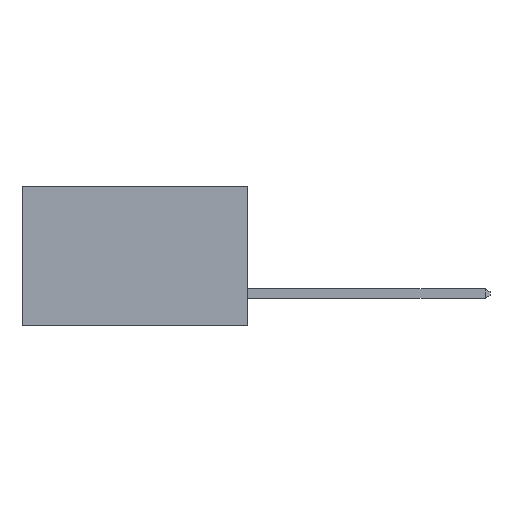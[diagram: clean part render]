
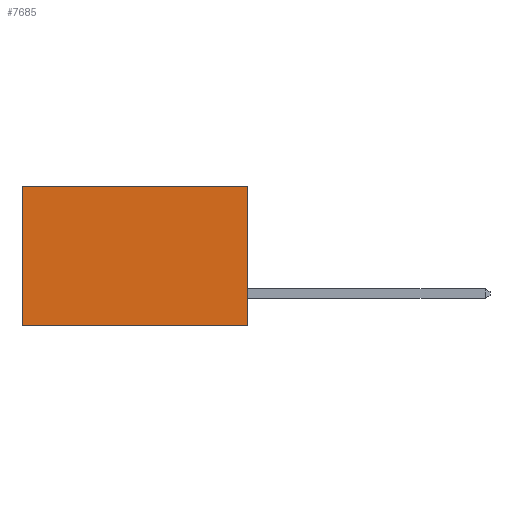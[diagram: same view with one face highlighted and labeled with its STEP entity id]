
A CAD part, left-side view. The second image highlights one B-rep face of the part: STEP entity #7685.
In plain terms, the highlighted planar face has unit normal (-1, 0, 0).
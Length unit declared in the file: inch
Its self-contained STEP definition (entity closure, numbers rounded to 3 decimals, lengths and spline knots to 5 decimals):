
#607 = VERTEX_POINT ( 'NONE', #7156 ) ;
#648 = CARTESIAN_POINT ( 'NONE',  ( 0.2615, 0., -0.37 ) ) ;
#774 = ORIENTED_EDGE ( 'NONE', *, *, #1543, .T. ) ;
#870 = VECTOR ( 'NONE', #1005, 39.37008 ) ;
#1005 = DIRECTION ( 'NONE',  ( 0., 0., -1. ) ) ;
#1362 = CARTESIAN_POINT ( 'NONE',  ( 0.2615, 0., -0.37 ) ) ;
#1461 = DIRECTION ( 'NONE',  ( 1., 0., 0. ) ) ;
#1543 = EDGE_CURVE ( 'NONE', #607, #3893, #1643, .T. ) ;
#1550 = DIRECTION ( 'NONE',  ( 0., 1., 0. ) ) ;
#1643 = LINE ( 'NONE', #3328, #7276 ) ;
#1658 = VECTOR ( 'NONE', #4089, 39.37008 ) ;
#2233 = DIRECTION ( 'NONE',  ( 0., 1., 0. ) ) ;
#2598 = ORIENTED_EDGE ( 'NONE', *, *, #7078, .F. ) ;
#3023 = EDGE_CURVE ( 'NONE', #607, #6880, #6800, .T. ) ;
#3256 = CARTESIAN_POINT ( 'NONE',  ( 0.2615, 0.6, 0. ) ) ;
#3328 = CARTESIAN_POINT ( 'NONE',  ( 0.2615, 0., 0. ) ) ;
#3733 = VECTOR ( 'NONE', #1550, 39.37008 ) ;
#3893 = VERTEX_POINT ( 'NONE', #3256 ) ;
#4089 = DIRECTION ( 'NONE',  ( 0., 0., -1. ) ) ;
#4316 = CARTESIAN_POINT ( 'NONE',  ( 0.2615, 0., -0.37 ) ) ;
#4859 = EDGE_CURVE ( 'NONE', #3893, #5587, #9327, .T. ) ;
#5212 = PLANE ( 'NONE',  #7702 ) ;
#5577 = CARTESIAN_POINT ( 'NONE',  ( 0.2615, 0.6, -0.37 ) ) ;
#5587 = VERTEX_POINT ( 'NONE', #8546 ) ;
#5809 = FACE_OUTER_BOUND ( 'NONE', #6011, .T. ) ;
#6011 = EDGE_LOOP ( 'NONE', ( #7914, #2598, #7823, #774 ) ) ;
#6637 = DIRECTION ( 'NONE',  ( 0., 0., -1. ) ) ;
#6707 = CARTESIAN_POINT ( 'NONE',  ( 0.2615, 0., -0.37 ) ) ;
#6800 = LINE ( 'NONE', #1362, #870 ) ;
#6880 = VERTEX_POINT ( 'NONE', #4316 ) ;
#7078 = EDGE_CURVE ( 'NONE', #6880, #5587, #7365, .T. ) ;
#7156 = CARTESIAN_POINT ( 'NONE',  ( 0.2615, 0., 0. ) ) ;
#7276 = VECTOR ( 'NONE', #2233, 39.37008 ) ;
#7365 = LINE ( 'NONE', #6707, #3733 ) ;
#7685 = ADVANCED_FACE ( 'NONE', ( #5809 ), #5212, .F. ) ;
#7702 = AXIS2_PLACEMENT_3D ( 'NONE', #648, #1461, #6637 ) ;
#7823 = ORIENTED_EDGE ( 'NONE', *, *, #3023, .F. ) ;
#7914 = ORIENTED_EDGE ( 'NONE', *, *, #4859, .T. ) ;
#8546 = CARTESIAN_POINT ( 'NONE',  ( 0.2615, 0.6, -0.37 ) ) ;
#9327 = LINE ( 'NONE', #5577, #1658 ) ;
